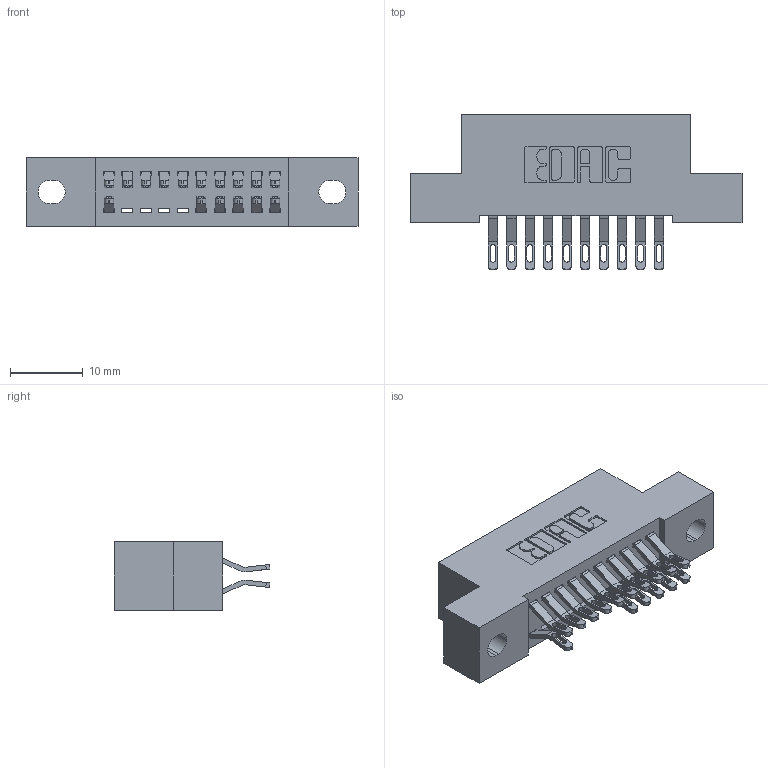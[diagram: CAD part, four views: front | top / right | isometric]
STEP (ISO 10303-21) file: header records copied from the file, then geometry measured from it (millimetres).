
FILE_DESCRIPTION (( 'STEP AP203' ), '1' );
FILE_NAME ('392-020-555-202.STEP', '2018-08-15T07:01:09', ( '' ), ( '' ), 'SwSTEP 2.0', 'SolidWorks 2016', '' );
FILE_SCHEMA (( 'CONFIG_CONTROL_DESIGN' ));
Length unit declared in the file: inch
Products named in the file (3): 342 Part_.128 Slot; 345-292-001_555 Tail; 392-020-555-202
Assembly tree (17 placements, depth 2):
  392-020-555-202
    342 Part_.128 Slot
    345-292-001_555 Tail  x16
Bounding box: 45.72 x 21.47 x 9.4 mm (x, y, z)
Volume: 3912.8 mm3; surface area: 5295.9 mm2
Topology: 17 solids, 17 shells, 1066 faces, 3323 edges, 2214 vertices
Faces by surface type: plane 638, cylinder 428
Entity records: 10773 total; most frequent: CARTESIAN_POINT 1876, ORIENTED_EDGE 1786, DIRECTION 1625, EDGE_CURVE 893, LINE 745, VECTOR 745, VERTEX_POINT 594, AXIS2_PLACEMENT_3D 440
